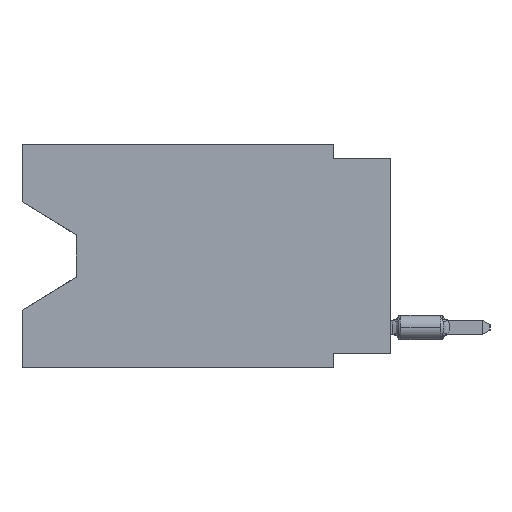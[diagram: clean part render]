
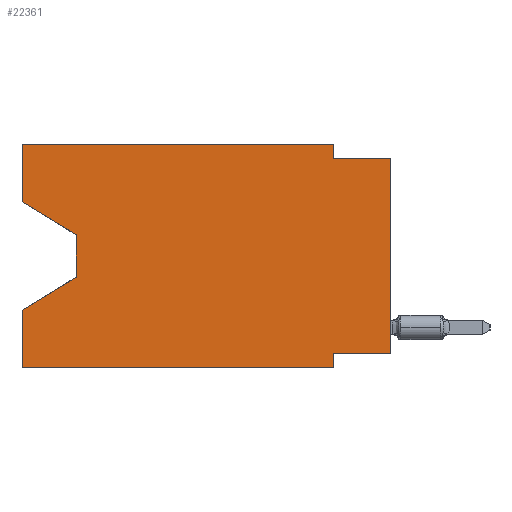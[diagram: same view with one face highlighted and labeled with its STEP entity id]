
A CAD part, left-side view. The second image highlights one B-rep face of the part: STEP entity #22361.
In plain terms, the highlighted planar face has unit normal (-1, 0, 0).
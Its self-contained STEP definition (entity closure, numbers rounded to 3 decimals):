
#190 = ORIENTED_EDGE ( 'NONE', *, *, #2646, .F. ) ;
#699 = CARTESIAN_POINT ( 'NONE',  ( 0., 16.383, -2.546 ) ) ;
#1329 = VECTOR ( 'NONE', #17074, 1000. ) ;
#1969 = EDGE_CURVE ( 'NONE', #22630, #2022, #18088, .T. ) ;
#2022 = VERTEX_POINT ( 'NONE', #2748 ) ;
#2646 = EDGE_CURVE ( 'NONE', #5528, #17947, #15058, .T. ) ;
#2735 = VECTOR ( 'NONE', #36067, 1000. ) ;
#2748 = CARTESIAN_POINT ( 'NONE',  ( 0., 16.383, -7.36 ) ) ;
#2896 = CARTESIAN_POINT ( 'NONE',  ( 0., 2.54, -9.271 ) ) ;
#2920 = ORIENTED_EDGE ( 'NONE', *, *, #5124, .F. ) ;
#3293 = ORIENTED_EDGE ( 'NONE', *, *, #12849, .F. ) ;
#3702 = CARTESIAN_POINT ( 'NONE',  ( 0., 0., -0.635 ) ) ;
#4225 = VERTEX_POINT ( 'NONE', #5368 ) ;
#4409 = VERTEX_POINT ( 'NONE', #32171 ) ;
#4550 = CARTESIAN_POINT ( 'NONE',  ( 0., 16.383, -9.906 ) ) ;
#4710 = LINE ( 'NONE', #23707, #11723 ) ;
#4938 = ORIENTED_EDGE ( 'NONE', *, *, #19839, .T. ) ;
#4990 = EDGE_CURVE ( 'NONE', #31690, #4409, #23277, .T. ) ;
#5124 = EDGE_CURVE ( 'NONE', #17947, #12557, #29295, .T. ) ;
#5368 = CARTESIAN_POINT ( 'NONE',  ( 0., 16.383, -2.546 ) ) ;
#5528 = VERTEX_POINT ( 'NONE', #18617 ) ;
#5585 = ORIENTED_EDGE ( 'NONE', *, *, #1969, .T. ) ;
#6692 = LINE ( 'NONE', #7028, #26301 ) ;
#6993 = LINE ( 'NONE', #18134, #13268 ) ;
#7028 = CARTESIAN_POINT ( 'NONE',  ( 0., 0., 0. ) ) ;
#7725 = LINE ( 'NONE', #27433, #21848 ) ;
#8856 = VERTEX_POINT ( 'NONE', #4550 ) ;
#11024 = ORIENTED_EDGE ( 'NONE', *, *, #19573, .T. ) ;
#11723 = VECTOR ( 'NONE', #26796, 1000. ) ;
#11984 = DIRECTION ( 'NONE',  ( 0., -1., 0. ) ) ;
#12160 = LINE ( 'NONE', #19996, #1329 ) ;
#12258 = VECTOR ( 'NONE', #31856, 1000. ) ;
#12557 = VERTEX_POINT ( 'NONE', #33309 ) ;
#12849 = EDGE_CURVE ( 'NONE', #4409, #21945, #6993, .T. ) ;
#13041 = CARTESIAN_POINT ( 'NONE',  ( 0., 16.383, 0. ) ) ;
#13268 = VECTOR ( 'NONE', #15217, 1000. ) ;
#15058 = LINE ( 'NONE', #19983, #12258 ) ;
#15217 = DIRECTION ( 'NONE',  ( 0., 0., -1. ) ) ;
#15221 = ORIENTED_EDGE ( 'NONE', *, *, #21545, .F. ) ;
#15290 = DIRECTION ( 'NONE',  ( 0., -0.855, -0.519 ) ) ;
#15296 = VECTOR ( 'NONE', #32898, 1000. ) ;
#15962 = CARTESIAN_POINT ( 'NONE',  ( 0., 13.97, -4.013 ) ) ;
#16104 = DIRECTION ( 'NONE',  ( 0., 0., -1. ) ) ;
#16631 = CARTESIAN_POINT ( 'NONE',  ( 0., 0., -0.635 ) ) ;
#16714 = CARTESIAN_POINT ( 'NONE',  ( 0., 16.383, 0. ) ) ;
#17074 = DIRECTION ( 'NONE',  ( 0., 0., 1. ) ) ;
#17947 = VERTEX_POINT ( 'NONE', #2896 ) ;
#18088 = LINE ( 'NONE', #26307, #28204 ) ;
#18134 = CARTESIAN_POINT ( 'NONE',  ( 0., 2.54, 0. ) ) ;
#18617 = CARTESIAN_POINT ( 'NONE',  ( 0., 0., -9.271 ) ) ;
#19090 = LINE ( 'NONE', #32796, #2735 ) ;
#19188 = CARTESIAN_POINT ( 'NONE',  ( 0., 2.54, -9.906 ) ) ;
#19573 = EDGE_CURVE ( 'NONE', #5528, #33099, #6692, .T. ) ;
#19662 = CARTESIAN_POINT ( 'NONE',  ( 0., 2.54, -0.635 ) ) ;
#19839 = EDGE_CURVE ( 'NONE', #4225, #34125, #25685, .T. ) ;
#19857 = AXIS2_PLACEMENT_3D ( 'NONE', #16714, #27689, #27848 ) ;
#19983 = CARTESIAN_POINT ( 'NONE',  ( 0., 0., -9.271 ) ) ;
#19996 = CARTESIAN_POINT ( 'NONE',  ( 0., 16.383, 0. ) ) ;
#20430 = ORIENTED_EDGE ( 'NONE', *, *, #32603, .F. ) ;
#21278 = DIRECTION ( 'NONE',  ( 0., 0., 1. ) ) ;
#21545 = EDGE_CURVE ( 'NONE', #4225, #31690, #12160, .T. ) ;
#21848 = VECTOR ( 'NONE', #23984, 1000. ) ;
#21945 = VERTEX_POINT ( 'NONE', #19662 ) ;
#22278 = VECTOR ( 'NONE', #16104, 1000. ) ;
#22361 = ADVANCED_FACE ( 'NONE', ( #22547 ), #30401, .F. ) ;
#22547 = FACE_OUTER_BOUND ( 'NONE', #25156, .T. ) ;
#22630 = VERTEX_POINT ( 'NONE', #27098 ) ;
#23277 = LINE ( 'NONE', #34807, #29848 ) ;
#23707 = CARTESIAN_POINT ( 'NONE',  ( 0., 13.97, -4.013 ) ) ;
#23984 = DIRECTION ( 'NONE',  ( 0., -1., 0. ) ) ;
#25156 = EDGE_LOOP ( 'NONE', ( #4938, #27898, #5585, #20430, #26122, #2920, #190, #11024, #25463, #3293, #31773, #15221 ) ) ;
#25463 = ORIENTED_EDGE ( 'NONE', *, *, #34698, .F. ) ;
#25685 = LINE ( 'NONE', #699, #32723 ) ;
#25773 = EDGE_CURVE ( 'NONE', #34125, #22630, #4710, .T. ) ;
#26122 = ORIENTED_EDGE ( 'NONE', *, *, #30057, .T. ) ;
#26301 = VECTOR ( 'NONE', #21278, 1000. ) ;
#26307 = CARTESIAN_POINT ( 'NONE',  ( 0., 13.97, -5.893 ) ) ;
#26796 = DIRECTION ( 'NONE',  ( 0., 0., -1. ) ) ;
#27098 = CARTESIAN_POINT ( 'NONE',  ( 0., 13.97, -5.893 ) ) ;
#27394 = LINE ( 'NONE', #16631, #15296 ) ;
#27433 = CARTESIAN_POINT ( 'NONE',  ( 0., 16.383, -9.906 ) ) ;
#27689 = DIRECTION ( 'NONE',  ( 1., 0., 0. ) ) ;
#27848 = DIRECTION ( 'NONE',  ( 0., 0., -1. ) ) ;
#27898 = ORIENTED_EDGE ( 'NONE', *, *, #25773, .T. ) ;
#28204 = VECTOR ( 'NONE', #29427, 1000. ) ;
#29295 = LINE ( 'NONE', #19188, #22278 ) ;
#29427 = DIRECTION ( 'NONE',  ( 0., 0.855, -0.519 ) ) ;
#29848 = VECTOR ( 'NONE', #11984, 1000. ) ;
#30057 = EDGE_CURVE ( 'NONE', #8856, #12557, #7725, .T. ) ;
#30401 = PLANE ( 'NONE',  #19857 ) ;
#31690 = VERTEX_POINT ( 'NONE', #13041 ) ;
#31773 = ORIENTED_EDGE ( 'NONE', *, *, #4990, .F. ) ;
#31856 = DIRECTION ( 'NONE',  ( 0., 1., 0. ) ) ;
#32171 = CARTESIAN_POINT ( 'NONE',  ( 0., 2.54, 0. ) ) ;
#32603 = EDGE_CURVE ( 'NONE', #8856, #2022, #19090, .T. ) ;
#32723 = VECTOR ( 'NONE', #15290, 1000. ) ;
#32796 = CARTESIAN_POINT ( 'NONE',  ( 0., 16.383, 0. ) ) ;
#32898 = DIRECTION ( 'NONE',  ( 0., -1., 0. ) ) ;
#33099 = VERTEX_POINT ( 'NONE', #3702 ) ;
#33309 = CARTESIAN_POINT ( 'NONE',  ( 0., 2.54, -9.906 ) ) ;
#34125 = VERTEX_POINT ( 'NONE', #15962 ) ;
#34698 = EDGE_CURVE ( 'NONE', #21945, #33099, #27394, .T. ) ;
#34807 = CARTESIAN_POINT ( 'NONE',  ( 0., 16.383, 0. ) ) ;
#36067 = DIRECTION ( 'NONE',  ( 0., 0., 1. ) ) ;
